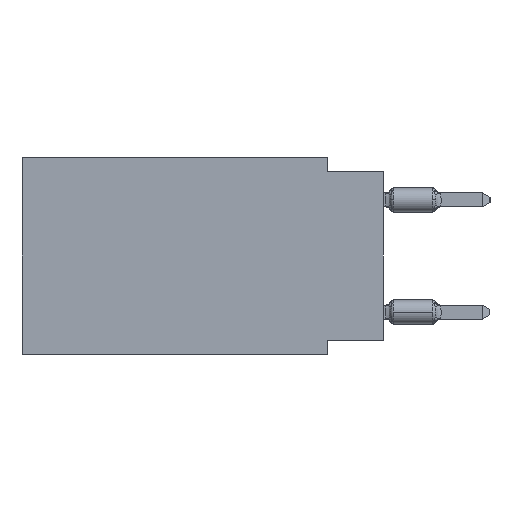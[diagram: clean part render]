
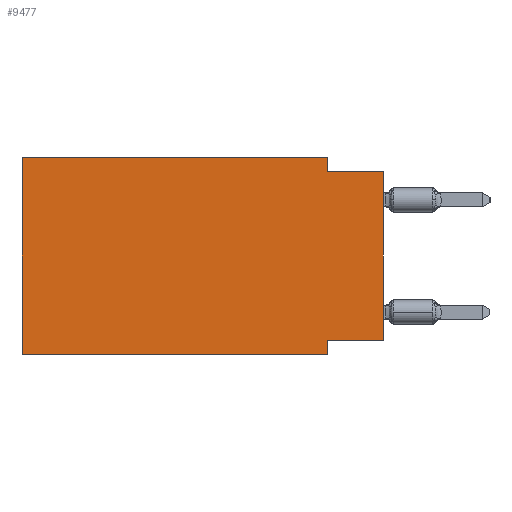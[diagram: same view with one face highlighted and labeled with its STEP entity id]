
A CAD part, left-side view. The second image highlights one B-rep face of the part: STEP entity #9477.
In plain terms, the highlighted planar face has unit normal (-1, 0, 0).
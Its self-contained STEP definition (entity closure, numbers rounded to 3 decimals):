
#500 = EDGE_CURVE ( 'NONE', #9694, #30960, #18049, .T. ) ;
#1160 = CARTESIAN_POINT ( 'NONE',  ( 0., 2.54, 0. ) ) ;
#2189 = VERTEX_POINT ( 'NONE', #23725 ) ;
#2615 = CARTESIAN_POINT ( 'NONE',  ( 0., 2.54, 0. ) ) ;
#3454 = VECTOR ( 'NONE', #18995, 1000. ) ;
#3594 = EDGE_CURVE ( 'NONE', #30960, #2189, #29322, .T. ) ;
#4352 = VECTOR ( 'NONE', #10129, 1000. ) ;
#4643 = VECTOR ( 'NONE', #8156, 1000. ) ;
#5336 = CARTESIAN_POINT ( 'NONE',  ( 0., 0., -0.635 ) ) ;
#5338 = VERTEX_POINT ( 'NONE', #14388 ) ;
#5520 = EDGE_CURVE ( 'NONE', #29353, #18528, #22724, .T. ) ;
#8006 = VECTOR ( 'NONE', #20652, 1000. ) ;
#8156 = DIRECTION ( 'NONE',  ( 0., -1., 0. ) ) ;
#8454 = VERTEX_POINT ( 'NONE', #2615 ) ;
#9477 = ADVANCED_FACE ( 'NONE', ( #21036 ), #21513, .F. ) ;
#9675 = ORIENTED_EDGE ( 'NONE', *, *, #29632, .F. ) ;
#9694 = VERTEX_POINT ( 'NONE', #14788 ) ;
#10129 = DIRECTION ( 'NONE',  ( 0., -1., 0. ) ) ;
#10883 = AXIS2_PLACEMENT_3D ( 'NONE', #16603, #23324, #26586 ) ;
#12125 = VERTEX_POINT ( 'NONE', #19186 ) ;
#12288 = ORIENTED_EDGE ( 'NONE', *, *, #30627, .T. ) ;
#12478 = EDGE_CURVE ( 'NONE', #8454, #29353, #29150, .T. ) ;
#12567 = ORIENTED_EDGE ( 'NONE', *, *, #20794, .T. ) ;
#12577 = CARTESIAN_POINT ( 'NONE',  ( 0., 2.54, -8.255 ) ) ;
#12612 = DIRECTION ( 'NONE',  ( 0., -1., 0. ) ) ;
#12849 = VECTOR ( 'NONE', #16558, 1000. ) ;
#12909 = ORIENTED_EDGE ( 'NONE', *, *, #5520, .F. ) ;
#12913 = LINE ( 'NONE', #20439, #4643 ) ;
#13397 = ORIENTED_EDGE ( 'NONE', *, *, #17703, .F. ) ;
#13699 = VECTOR ( 'NONE', #17833, 1000. ) ;
#14388 = CARTESIAN_POINT ( 'NONE',  ( 0., 16.383, -8.89 ) ) ;
#14788 = CARTESIAN_POINT ( 'NONE',  ( 0., 0., -8.255 ) ) ;
#15419 = LINE ( 'NONE', #18039, #19879 ) ;
#16558 = DIRECTION ( 'NONE',  ( 0., 0., -1. ) ) ;
#16603 = CARTESIAN_POINT ( 'NONE',  ( 0., 16.383, 0. ) ) ;
#17703 = EDGE_CURVE ( 'NONE', #12125, #8454, #12913, .T. ) ;
#17833 = DIRECTION ( 'NONE',  ( 0., 0., 1. ) ) ;
#18039 = CARTESIAN_POINT ( 'NONE',  ( 0., 0., 0. ) ) ;
#18049 = LINE ( 'NONE', #18367, #8006 ) ;
#18367 = CARTESIAN_POINT ( 'NONE',  ( 0., 0., -8.255 ) ) ;
#18528 = VERTEX_POINT ( 'NONE', #5336 ) ;
#18961 = VECTOR ( 'NONE', #12612, 1000. ) ;
#18995 = DIRECTION ( 'NONE',  ( 0., 0., -1. ) ) ;
#19186 = CARTESIAN_POINT ( 'NONE',  ( 0., 16.383, 0. ) ) ;
#19619 = LINE ( 'NONE', #29949, #13699 ) ;
#19879 = VECTOR ( 'NONE', #28954, 1000. ) ;
#19953 = ORIENTED_EDGE ( 'NONE', *, *, #500, .F. ) ;
#20439 = CARTESIAN_POINT ( 'NONE',  ( 0., 16.383, 0. ) ) ;
#20652 = DIRECTION ( 'NONE',  ( 0., 1., 0. ) ) ;
#20794 = EDGE_CURVE ( 'NONE', #9694, #18528, #15419, .T. ) ;
#21036 = FACE_OUTER_BOUND ( 'NONE', #29396, .T. ) ;
#21124 = CARTESIAN_POINT ( 'NONE',  ( 0., 2.54, -0.635 ) ) ;
#21513 = PLANE ( 'NONE',  #10883 ) ;
#21844 = ORIENTED_EDGE ( 'NONE', *, *, #3594, .F. ) ;
#22724 = LINE ( 'NONE', #32228, #4352 ) ;
#23077 = CARTESIAN_POINT ( 'NONE',  ( 0., 16.383, -8.89 ) ) ;
#23324 = DIRECTION ( 'NONE',  ( 1., 0., 0. ) ) ;
#23725 = CARTESIAN_POINT ( 'NONE',  ( 0., 2.54, -8.89 ) ) ;
#25058 = LINE ( 'NONE', #23077, #18961 ) ;
#26382 = CARTESIAN_POINT ( 'NONE',  ( 0., 2.54, -8.89 ) ) ;
#26586 = DIRECTION ( 'NONE',  ( 0., 0., -1. ) ) ;
#28954 = DIRECTION ( 'NONE',  ( 0., 0., 1. ) ) ;
#29150 = LINE ( 'NONE', #1160, #3454 ) ;
#29322 = LINE ( 'NONE', #26382, #12849 ) ;
#29353 = VERTEX_POINT ( 'NONE', #21124 ) ;
#29396 = EDGE_LOOP ( 'NONE', ( #12567, #12909, #29768, #13397, #9675, #12288, #21844, #19953 ) ) ;
#29632 = EDGE_CURVE ( 'NONE', #5338, #12125, #19619, .T. ) ;
#29768 = ORIENTED_EDGE ( 'NONE', *, *, #12478, .F. ) ;
#29949 = CARTESIAN_POINT ( 'NONE',  ( 0., 16.383, 0. ) ) ;
#30627 = EDGE_CURVE ( 'NONE', #5338, #2189, #25058, .T. ) ;
#30960 = VERTEX_POINT ( 'NONE', #12577 ) ;
#32228 = CARTESIAN_POINT ( 'NONE',  ( 0., 0., -0.635 ) ) ;
